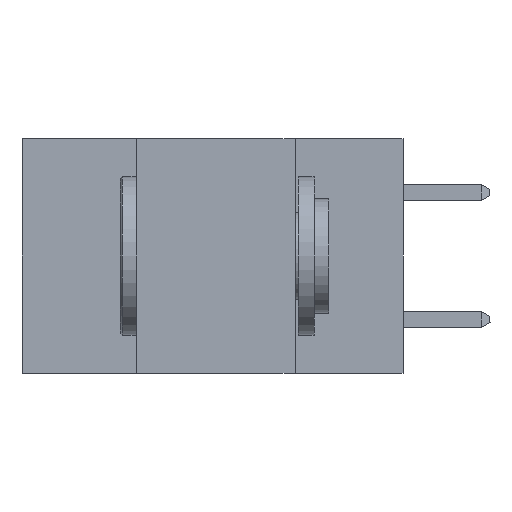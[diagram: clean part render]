
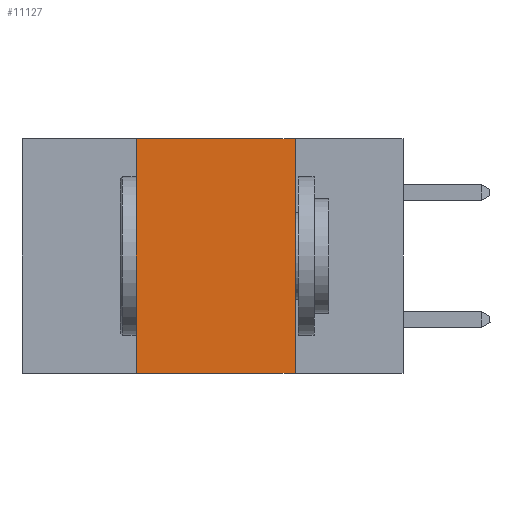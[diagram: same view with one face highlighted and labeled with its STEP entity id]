
A CAD part, left-side view. The second image highlights one B-rep face of the part: STEP entity #11127.
In plain terms, the highlighted planar face has unit normal (-1, 0, 0).
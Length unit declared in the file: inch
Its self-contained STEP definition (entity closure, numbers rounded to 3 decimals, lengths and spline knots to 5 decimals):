
#6 = DIRECTION ( 'NONE',  ( 1., 0., 0. ) ) ;
#127 = CARTESIAN_POINT ( 'NONE',  ( 0., 0.17, 0. ) ) ;
#1124 = AXIS2_PLACEMENT_3D ( 'NONE', #9693, #6, #5464 ) ;
#1474 = LINE ( 'NONE', #2582, #10478 ) ;
#1694 = CARTESIAN_POINT ( 'NONE',  ( 0., 0.17, -0.37 ) ) ;
#2382 = ORIENTED_EDGE ( 'NONE', *, *, #4146, .F. ) ;
#2582 = CARTESIAN_POINT ( 'NONE',  ( 0., 0.6, -0.37 ) ) ;
#2639 = CARTESIAN_POINT ( 'NONE',  ( 0., 0.42, -0.37 ) ) ;
#2948 = CARTESIAN_POINT ( 'NONE',  ( 0., 0.17, 0. ) ) ;
#3058 = LINE ( 'NONE', #7482, #4820 ) ;
#3396 = VERTEX_POINT ( 'NONE', #2639 ) ;
#3403 = VECTOR ( 'NONE', #12707, 39.37008 ) ;
#4146 = EDGE_CURVE ( 'NONE', #9389, #15426, #13059, .T. ) ;
#4820 = VECTOR ( 'NONE', #17312, 39.37008 ) ;
#5011 = LINE ( 'NONE', #11097, #6299 ) ;
#5342 = PLANE ( 'NONE',  #1124 ) ;
#5464 = DIRECTION ( 'NONE',  ( 0., 0., -1. ) ) ;
#6299 = VECTOR ( 'NONE', #12834, 39.37008 ) ;
#6753 = VERTEX_POINT ( 'NONE', #11327 ) ;
#7482 = CARTESIAN_POINT ( 'NONE',  ( 0., 0.6, 0. ) ) ;
#7796 = EDGE_LOOP ( 'NONE', ( #2382, #9103, #8861, #8784 ) ) ;
#8784 = ORIENTED_EDGE ( 'NONE', *, *, #12693, .T. ) ;
#8861 = ORIENTED_EDGE ( 'NONE', *, *, #11168, .F. ) ;
#9103 = ORIENTED_EDGE ( 'NONE', *, *, #17383, .F. ) ;
#9389 = VERTEX_POINT ( 'NONE', #2948 ) ;
#9693 = CARTESIAN_POINT ( 'NONE',  ( 0., 0.6, 0. ) ) ;
#10478 = VECTOR ( 'NONE', #15362, 39.37008 ) ;
#11097 = CARTESIAN_POINT ( 'NONE',  ( 0., 0.42, 0. ) ) ;
#11127 = ADVANCED_FACE ( 'NONE', ( #17526 ), #5342, .F. ) ;
#11168 = EDGE_CURVE ( 'NONE', #3396, #6753, #5011, .T. ) ;
#11327 = CARTESIAN_POINT ( 'NONE',  ( 0., 0.42, 0. ) ) ;
#12693 = EDGE_CURVE ( 'NONE', #3396, #15426, #1474, .T. ) ;
#12707 = DIRECTION ( 'NONE',  ( 0., 0., -1. ) ) ;
#12834 = DIRECTION ( 'NONE',  ( 0., 0., 1. ) ) ;
#13059 = LINE ( 'NONE', #127, #3403 ) ;
#15362 = DIRECTION ( 'NONE',  ( 0., -1., 0. ) ) ;
#15426 = VERTEX_POINT ( 'NONE', #1694 ) ;
#17312 = DIRECTION ( 'NONE',  ( 0., -1., 0. ) ) ;
#17383 = EDGE_CURVE ( 'NONE', #6753, #9389, #3058, .T. ) ;
#17526 = FACE_OUTER_BOUND ( 'NONE', #7796, .T. ) ;
